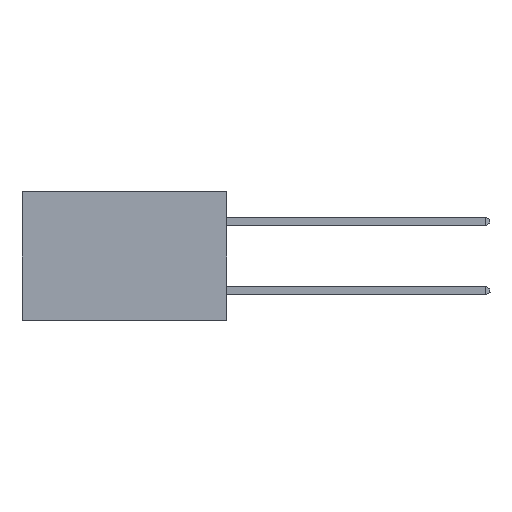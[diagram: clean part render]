
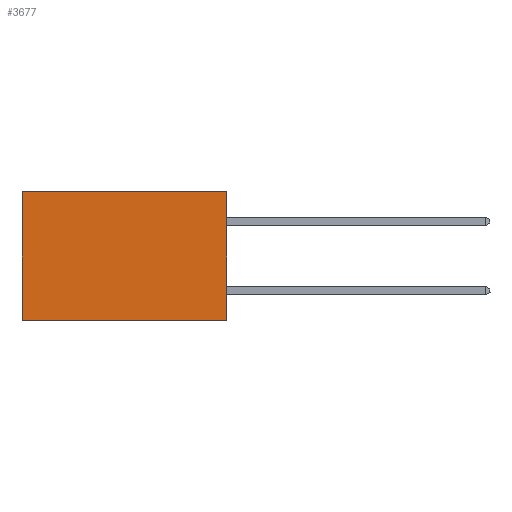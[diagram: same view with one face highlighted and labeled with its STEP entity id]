
A CAD part, left-side view. The second image highlights one B-rep face of the part: STEP entity #3677.
In plain terms, the highlighted planar face has unit normal (-1, 0, 0).
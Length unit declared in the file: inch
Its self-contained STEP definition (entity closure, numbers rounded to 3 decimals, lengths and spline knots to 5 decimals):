
#732 = EDGE_CURVE ( 'NONE', #18992, #6378, #4446, .T. ) ;
#824 = VECTOR ( 'NONE', #19300, 39.37008 ) ;
#1317 = EDGE_LOOP ( 'NONE', ( #19824, #3381, #19655, #19198 ) ) ;
#1852 = FACE_OUTER_BOUND ( 'NONE', #1317, .T. ) ;
#2315 = EDGE_CURVE ( 'NONE', #18019, #6378, #5116, .T. ) ;
#2350 = VERTEX_POINT ( 'NONE', #8769 ) ;
#2527 = CARTESIAN_POINT ( 'NONE',  ( 0.277, 0., -0.37 ) ) ;
#3100 = DIRECTION ( 'NONE',  ( 0., 1., 0. ) ) ;
#3381 = ORIENTED_EDGE ( 'NONE', *, *, #2315, .F. ) ;
#3677 = ADVANCED_FACE ( 'NONE', ( #1852 ), #18710, .F. ) ;
#4446 = LINE ( 'NONE', #9873, #17526 ) ;
#5116 = LINE ( 'NONE', #5837, #824 ) ;
#5837 = CARTESIAN_POINT ( 'NONE',  ( 0.277, 0., -0.37 ) ) ;
#5909 = CARTESIAN_POINT ( 'NONE',  ( 0.277, 0., -0.37 ) ) ;
#6378 = VERTEX_POINT ( 'NONE', #12258 ) ;
#7208 = DIRECTION ( 'NONE',  ( 0., 0., -1. ) ) ;
#7274 = VECTOR ( 'NONE', #3100, 39.37008 ) ;
#8769 = CARTESIAN_POINT ( 'NONE',  ( 0.277, 0., 0. ) ) ;
#9873 = CARTESIAN_POINT ( 'NONE',  ( 0.277, 0.59, -0.37 ) ) ;
#11486 = LINE ( 'NONE', #20323, #7274 ) ;
#12258 = CARTESIAN_POINT ( 'NONE',  ( 0.277, 0.59, -0.37 ) ) ;
#13626 = VECTOR ( 'NONE', #15390, 39.37008 ) ;
#15390 = DIRECTION ( 'NONE',  ( 0., 0., -1. ) ) ;
#16361 = EDGE_CURVE ( 'NONE', #2350, #18992, #11486, .T. ) ;
#16364 = AXIS2_PLACEMENT_3D ( 'NONE', #18939, #18707, #18644 ) ;
#17526 = VECTOR ( 'NONE', #7208, 39.37008 ) ;
#17782 = LINE ( 'NONE', #5909, #13626 ) ;
#17848 = CARTESIAN_POINT ( 'NONE',  ( 0.277, 0.59, 0. ) ) ;
#18019 = VERTEX_POINT ( 'NONE', #2527 ) ;
#18578 = EDGE_CURVE ( 'NONE', #2350, #18019, #17782, .T. ) ;
#18644 = DIRECTION ( 'NONE',  ( 0., 0., -1. ) ) ;
#18707 = DIRECTION ( 'NONE',  ( 1., 0., 0. ) ) ;
#18710 = PLANE ( 'NONE',  #16364 ) ;
#18939 = CARTESIAN_POINT ( 'NONE',  ( 0.277, 0., -0.37 ) ) ;
#18992 = VERTEX_POINT ( 'NONE', #17848 ) ;
#19198 = ORIENTED_EDGE ( 'NONE', *, *, #16361, .T. ) ;
#19300 = DIRECTION ( 'NONE',  ( 0., 1., 0. ) ) ;
#19655 = ORIENTED_EDGE ( 'NONE', *, *, #18578, .F. ) ;
#19824 = ORIENTED_EDGE ( 'NONE', *, *, #732, .T. ) ;
#20323 = CARTESIAN_POINT ( 'NONE',  ( 0.277, 0., 0. ) ) ;
